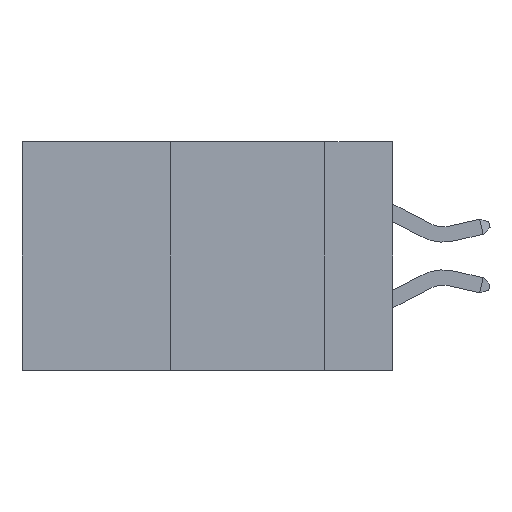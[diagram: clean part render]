
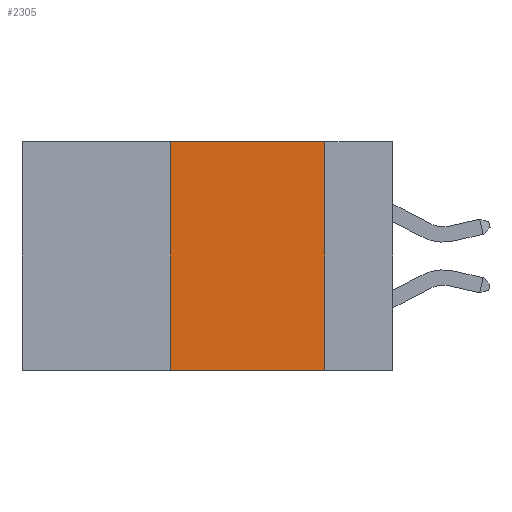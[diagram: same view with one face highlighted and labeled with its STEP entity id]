
A CAD part, left-side view. The second image highlights one B-rep face of the part: STEP entity #2305.
In plain terms, the highlighted planar face has unit normal (-1, 0, 0).
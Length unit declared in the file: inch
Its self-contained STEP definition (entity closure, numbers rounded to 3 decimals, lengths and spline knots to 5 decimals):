
#808 = VERTEX_POINT ( 'NONE', #4440 ) ;
#906 = EDGE_CURVE ( 'NONE', #2315, #6394, #3912, .T. ) ;
#1379 = EDGE_CURVE ( 'NONE', #808, #2315, #4069, .T. ) ;
#1497 = FACE_OUTER_BOUND ( 'NONE', #3808, .T. ) ;
#1554 = ORIENTED_EDGE ( 'NONE', *, *, #906, .F. ) ;
#1693 = CARTESIAN_POINT ( 'NONE',  ( 0., 0.6, -0.37 ) ) ;
#1974 = AXIS2_PLACEMENT_3D ( 'NONE', #4996, #10955, #2208 ) ;
#2015 = CARTESIAN_POINT ( 'NONE',  ( 0., 0.36, 0. ) ) ;
#2208 = DIRECTION ( 'NONE',  ( 0., 0., -1. ) ) ;
#2305 = ADVANCED_FACE ( 'NONE', ( #1497 ), #4832, .F. ) ;
#2315 = VERTEX_POINT ( 'NONE', #5653 ) ;
#2911 = EDGE_CURVE ( 'NONE', #10778, #6394, #4364, .T. ) ;
#3071 = DIRECTION ( 'NONE',  ( 0., -1., 0. ) ) ;
#3198 = DIRECTION ( 'NONE',  ( 0., 0., -1. ) ) ;
#3671 = LINE ( 'NONE', #2015, #9400 ) ;
#3808 = EDGE_LOOP ( 'NONE', ( #1554, #5491, #6950, #8544 ) ) ;
#3832 = EDGE_CURVE ( 'NONE', #10778, #808, #3671, .T. ) ;
#3912 = LINE ( 'NONE', #9930, #4839 ) ;
#4069 = LINE ( 'NONE', #6362, #6560 ) ;
#4245 = DIRECTION ( 'NONE',  ( 0., -1., 0. ) ) ;
#4364 = LINE ( 'NONE', #1693, #4979 ) ;
#4440 = CARTESIAN_POINT ( 'NONE',  ( 0., 0.36, 0. ) ) ;
#4832 = PLANE ( 'NONE',  #1974 ) ;
#4839 = VECTOR ( 'NONE', #3198, 39.37008 ) ;
#4979 = VECTOR ( 'NONE', #4245, 39.37008 ) ;
#4996 = CARTESIAN_POINT ( 'NONE',  ( 0., 0.6, 0. ) ) ;
#5292 = CARTESIAN_POINT ( 'NONE',  ( 0., 0.36, -0.37 ) ) ;
#5318 = CARTESIAN_POINT ( 'NONE',  ( 0., 0.11, -0.37 ) ) ;
#5491 = ORIENTED_EDGE ( 'NONE', *, *, #1379, .F. ) ;
#5653 = CARTESIAN_POINT ( 'NONE',  ( 0., 0.11, 0. ) ) ;
#6362 = CARTESIAN_POINT ( 'NONE',  ( 0., 0.6, 0. ) ) ;
#6394 = VERTEX_POINT ( 'NONE', #5318 ) ;
#6560 = VECTOR ( 'NONE', #3071, 39.37008 ) ;
#6950 = ORIENTED_EDGE ( 'NONE', *, *, #3832, .F. ) ;
#8544 = ORIENTED_EDGE ( 'NONE', *, *, #2911, .T. ) ;
#8839 = DIRECTION ( 'NONE',  ( 0., 0., 1. ) ) ;
#9400 = VECTOR ( 'NONE', #8839, 39.37008 ) ;
#9930 = CARTESIAN_POINT ( 'NONE',  ( 0., 0.11, 0. ) ) ;
#10778 = VERTEX_POINT ( 'NONE', #5292 ) ;
#10955 = DIRECTION ( 'NONE',  ( 1., 0., 0. ) ) ;
